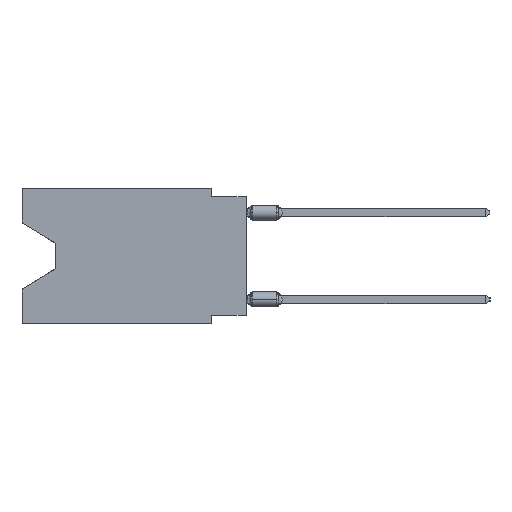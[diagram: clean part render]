
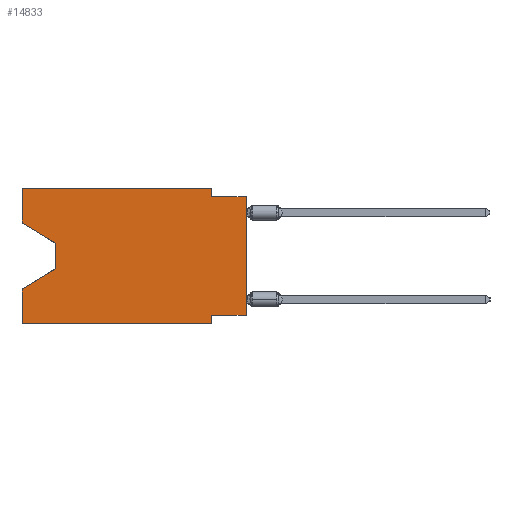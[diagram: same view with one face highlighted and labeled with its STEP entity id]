
A CAD part, left-side view. The second image highlights one B-rep face of the part: STEP entity #14833.
In plain terms, the highlighted planar face has unit normal (-1, 0, 0).
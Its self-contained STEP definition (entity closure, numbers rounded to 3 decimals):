
#132 = ORIENTED_EDGE ( 'NONE', *, *, #11569, .T. ) ;
#593 = VECTOR ( 'NONE', #7332, 1000. ) ;
#643 = ORIENTED_EDGE ( 'NONE', *, *, #32417, .T. ) ;
#1361 = EDGE_CURVE ( 'NONE', #33145, #5656, #26493, .T. ) ;
#1837 = CARTESIAN_POINT ( 'NONE',  ( 0., 0., -0.635 ) ) ;
#1938 = ORIENTED_EDGE ( 'NONE', *, *, #5462, .F. ) ;
#2176 = CARTESIAN_POINT ( 'NONE',  ( 0., 16.383, -7.36 ) ) ;
#2551 = VERTEX_POINT ( 'NONE', #3685 ) ;
#3016 = VERTEX_POINT ( 'NONE', #17621 ) ;
#3226 = ORIENTED_EDGE ( 'NONE', *, *, #14622, .F. ) ;
#3685 = CARTESIAN_POINT ( 'NONE',  ( 0., 16.383, -2.546 ) ) ;
#4575 = ORIENTED_EDGE ( 'NONE', *, *, #34299, .F. ) ;
#4681 = PLANE ( 'NONE',  #22363 ) ;
#5068 = VECTOR ( 'NONE', #25551, 1000. ) ;
#5462 = EDGE_CURVE ( 'NONE', #15642, #3016, #25301, .T. ) ;
#5656 = VERTEX_POINT ( 'NONE', #21552 ) ;
#5672 = VERTEX_POINT ( 'NONE', #2176 ) ;
#7119 = CARTESIAN_POINT ( 'NONE',  ( 0., 13.97, -5.893 ) ) ;
#7332 = DIRECTION ( 'NONE',  ( 0., -1., 0. ) ) ;
#7816 = VECTOR ( 'NONE', #18932, 1000. ) ;
#8042 = CARTESIAN_POINT ( 'NONE',  ( 0., 2.54, 0. ) ) ;
#8416 = VERTEX_POINT ( 'NONE', #15039 ) ;
#9039 = ORIENTED_EDGE ( 'NONE', *, *, #22241, .T. ) ;
#9790 = VECTOR ( 'NONE', #34201, 1000. ) ;
#10483 = LINE ( 'NONE', #27248, #593 ) ;
#11002 = CARTESIAN_POINT ( 'NONE',  ( 0., 16.383, 0. ) ) ;
#11422 = CARTESIAN_POINT ( 'NONE',  ( 0., 0., -9.271 ) ) ;
#11569 = EDGE_CURVE ( 'NONE', #2551, #26555, #23964, .T. ) ;
#12458 = VERTEX_POINT ( 'NONE', #16585 ) ;
#12894 = ORIENTED_EDGE ( 'NONE', *, *, #25903, .F. ) ;
#14024 = VECTOR ( 'NONE', #21280, 1000. ) ;
#14622 = EDGE_CURVE ( 'NONE', #15255, #12458, #31131, .T. ) ;
#14780 = VECTOR ( 'NONE', #36288, 1000. ) ;
#14807 = CARTESIAN_POINT ( 'NONE',  ( 0., 13.97, -4.013 ) ) ;
#14833 = ADVANCED_FACE ( 'NONE', ( #18454 ), #4681, .F. ) ;
#15039 = CARTESIAN_POINT ( 'NONE',  ( 0., 16.383, 0. ) ) ;
#15071 = DIRECTION ( 'NONE',  ( 0., 0., -1. ) ) ;
#15255 = VERTEX_POINT ( 'NONE', #18056 ) ;
#15642 = VERTEX_POINT ( 'NONE', #32162 ) ;
#16585 = CARTESIAN_POINT ( 'NONE',  ( 0., 2.54, -0.635 ) ) ;
#17025 = LINE ( 'NONE', #11422, #22881 ) ;
#17223 = EDGE_LOOP ( 'NONE', ( #132, #643, #9039, #27781, #25226, #1938, #28621, #20792, #12894, #3226, #4575, #28172 ) ) ;
#17371 = DIRECTION ( 'NONE',  ( 0., 0., 1. ) ) ;
#17602 = CARTESIAN_POINT ( 'NONE',  ( 0., 0., -9.271 ) ) ;
#17621 = CARTESIAN_POINT ( 'NONE',  ( 0., 2.54, -9.906 ) ) ;
#18056 = CARTESIAN_POINT ( 'NONE',  ( 0., 2.54, 0. ) ) ;
#18454 = FACE_OUTER_BOUND ( 'NONE', #17223, .T. ) ;
#18932 = DIRECTION ( 'NONE',  ( 0., -0.855, -0.519 ) ) ;
#19324 = VECTOR ( 'NONE', #27707, 1000. ) ;
#19833 = VERTEX_POINT ( 'NONE', #25929 ) ;
#20058 = LINE ( 'NONE', #33651, #9790 ) ;
#20341 = EDGE_CURVE ( 'NONE', #33145, #15642, #17025, .T. ) ;
#20792 = ORIENTED_EDGE ( 'NONE', *, *, #1361, .T. ) ;
#21280 = DIRECTION ( 'NONE',  ( 0., 0.855, -0.519 ) ) ;
#21530 = EDGE_CURVE ( 'NONE', #19833, #3016, #20058, .T. ) ;
#21552 = CARTESIAN_POINT ( 'NONE',  ( 0., 0., -0.635 ) ) ;
#22131 = LINE ( 'NONE', #1837, #19324 ) ;
#22241 = EDGE_CURVE ( 'NONE', #28942, #5672, #32809, .T. ) ;
#22363 = AXIS2_PLACEMENT_3D ( 'NONE', #29807, #33162, #32434 ) ;
#22844 = CARTESIAN_POINT ( 'NONE',  ( 0., 13.97, -5.893 ) ) ;
#22881 = VECTOR ( 'NONE', #31532, 1000. ) ;
#23107 = CARTESIAN_POINT ( 'NONE',  ( 0., 13.97, -4.013 ) ) ;
#23650 = VECTOR ( 'NONE', #34237, 1000. ) ;
#23964 = LINE ( 'NONE', #24516, #7816 ) ;
#24516 = CARTESIAN_POINT ( 'NONE',  ( 0., 16.383, -2.546 ) ) ;
#24940 = CARTESIAN_POINT ( 'NONE',  ( 0., 0., 0. ) ) ;
#25226 = ORIENTED_EDGE ( 'NONE', *, *, #21530, .T. ) ;
#25301 = LINE ( 'NONE', #34421, #25699 ) ;
#25384 = LINE ( 'NONE', #36737, #29186 ) ;
#25551 = DIRECTION ( 'NONE',  ( 0., 0., -1. ) ) ;
#25699 = VECTOR ( 'NONE', #28278, 1000. ) ;
#25903 = EDGE_CURVE ( 'NONE', #12458, #5656, #22131, .T. ) ;
#25929 = CARTESIAN_POINT ( 'NONE',  ( 0., 16.383, -9.906 ) ) ;
#26493 = LINE ( 'NONE', #24940, #14780 ) ;
#26555 = VERTEX_POINT ( 'NONE', #14807 ) ;
#27248 = CARTESIAN_POINT ( 'NONE',  ( 0., 16.383, 0. ) ) ;
#27707 = DIRECTION ( 'NONE',  ( 0., -1., 0. ) ) ;
#27781 = ORIENTED_EDGE ( 'NONE', *, *, #28625, .F. ) ;
#28172 = ORIENTED_EDGE ( 'NONE', *, *, #35497, .F. ) ;
#28198 = VECTOR ( 'NONE', #15071, 1000. ) ;
#28278 = DIRECTION ( 'NONE',  ( 0., 0., -1. ) ) ;
#28621 = ORIENTED_EDGE ( 'NONE', *, *, #20341, .F. ) ;
#28625 = EDGE_CURVE ( 'NONE', #19833, #5672, #36514, .T. ) ;
#28942 = VERTEX_POINT ( 'NONE', #22844 ) ;
#29186 = VECTOR ( 'NONE', #17371, 1000. ) ;
#29807 = CARTESIAN_POINT ( 'NONE',  ( 0., 16.383, 0. ) ) ;
#31131 = LINE ( 'NONE', #8042, #5068 ) ;
#31532 = DIRECTION ( 'NONE',  ( 0., 1., 0. ) ) ;
#32162 = CARTESIAN_POINT ( 'NONE',  ( 0., 2.54, -9.271 ) ) ;
#32417 = EDGE_CURVE ( 'NONE', #26555, #28942, #34996, .T. ) ;
#32434 = DIRECTION ( 'NONE',  ( 0., 0., -1. ) ) ;
#32809 = LINE ( 'NONE', #7119, #14024 ) ;
#33145 = VERTEX_POINT ( 'NONE', #17602 ) ;
#33162 = DIRECTION ( 'NONE',  ( 1., 0., 0. ) ) ;
#33651 = CARTESIAN_POINT ( 'NONE',  ( 0., 16.383, -9.906 ) ) ;
#34201 = DIRECTION ( 'NONE',  ( 0., -1., 0. ) ) ;
#34237 = DIRECTION ( 'NONE',  ( 0., 0., 1. ) ) ;
#34299 = EDGE_CURVE ( 'NONE', #8416, #15255, #10483, .T. ) ;
#34421 = CARTESIAN_POINT ( 'NONE',  ( 0., 2.54, -9.906 ) ) ;
#34996 = LINE ( 'NONE', #23107, #28198 ) ;
#35497 = EDGE_CURVE ( 'NONE', #2551, #8416, #25384, .T. ) ;
#36288 = DIRECTION ( 'NONE',  ( 0., 0., 1. ) ) ;
#36514 = LINE ( 'NONE', #11002, #23650 ) ;
#36737 = CARTESIAN_POINT ( 'NONE',  ( 0., 16.383, 0. ) ) ;
